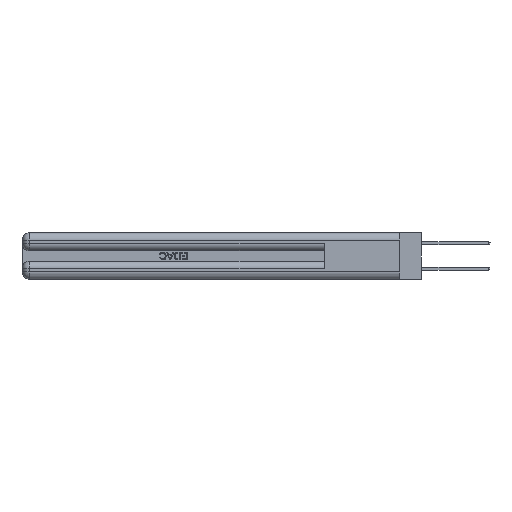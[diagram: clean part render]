
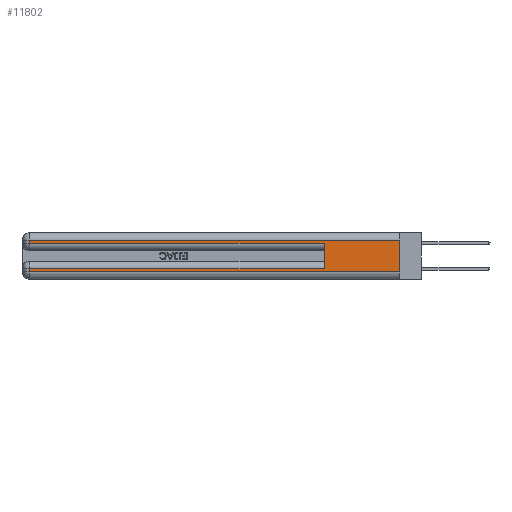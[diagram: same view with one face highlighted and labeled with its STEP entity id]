
A CAD part, left-side view. The second image highlights one B-rep face of the part: STEP entity #11802.
In plain terms, the highlighted planar face has unit normal (-1, 0, 0).
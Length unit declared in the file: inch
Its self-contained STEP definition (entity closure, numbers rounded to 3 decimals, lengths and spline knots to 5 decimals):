
#711 = DIRECTION ( 'NONE',  ( 0., -1., 0. ) ) ;
#1055 = VECTOR ( 'NONE', #711, 39.37008 ) ;
#1711 = EDGE_CURVE ( 'NONE', #34496, #46931, #38199, .T. ) ;
#2242 = DIRECTION ( 'NONE',  ( 1., 0., 0. ) ) ;
#2792 = VERTEX_POINT ( 'NONE', #23852 ) ;
#2886 = DIRECTION ( 'NONE',  ( 0., -1., 0. ) ) ;
#3246 = ORIENTED_EDGE ( 'NONE', *, *, #6224, .T. ) ;
#3574 = EDGE_CURVE ( 'NONE', #2792, #42154, #43149, .T. ) ;
#4545 = LINE ( 'NONE', #44220, #30268 ) ;
#6024 = CARTESIAN_POINT ( 'NONE',  ( 0., 0.6, 0.145 ) ) ;
#6224 = EDGE_CURVE ( 'NONE', #8268, #46931, #25648, .T. ) ;
#7801 = VECTOR ( 'NONE', #20749, 39.37008 ) ;
#8268 = VERTEX_POINT ( 'NONE', #28510 ) ;
#10424 = EDGE_LOOP ( 'NONE', ( #37490, #43085, #34774, #3246, #31566, #31514, #31092, #27374 ) ) ;
#10756 = CARTESIAN_POINT ( 'NONE',  ( 0., 2.94, 0.085 ) ) ;
#11802 = ADVANCED_FACE ( 'NONE', ( #24345 ), #24091, .F. ) ;
#12672 = VERTEX_POINT ( 'NONE', #22584 ) ;
#13892 = VECTOR ( 'NONE', #20384, 39.37008 ) ;
#14137 = VECTOR ( 'NONE', #45465, 39.37008 ) ;
#15295 = LINE ( 'NONE', #41638, #14137 ) ;
#15775 = VECTOR ( 'NONE', #31794, 39.37008 ) ;
#15935 = VECTOR ( 'NONE', #2886, 39.37008 ) ;
#18915 = CARTESIAN_POINT ( 'NONE',  ( 0., 0., 0.06 ) ) ;
#20384 = DIRECTION ( 'NONE',  ( 0., 1., 0. ) ) ;
#20749 = DIRECTION ( 'NONE',  ( 0., 0., 1. ) ) ;
#22584 = CARTESIAN_POINT ( 'NONE',  ( 0., 2.94, 0.06 ) ) ;
#22825 = EDGE_CURVE ( 'NONE', #42154, #8268, #15295, .T. ) ;
#23852 = CARTESIAN_POINT ( 'NONE',  ( 0., 0., 0.31 ) ) ;
#24046 = CARTESIAN_POINT ( 'NONE',  ( 0., 0., 0.31 ) ) ;
#24083 = CARTESIAN_POINT ( 'NONE',  ( 0., 0., 0.06 ) ) ;
#24091 = PLANE ( 'NONE',  #29608 ) ;
#24345 = FACE_OUTER_BOUND ( 'NONE', #10424, .T. ) ;
#25014 = CARTESIAN_POINT ( 'NONE',  ( 0., 0.6, 0.285 ) ) ;
#25648 = LINE ( 'NONE', #28411, #15935 ) ;
#27370 = EDGE_CURVE ( 'NONE', #34496, #30808, #35233, .T. ) ;
#27374 = ORIENTED_EDGE ( 'NONE', *, *, #32961, .T. ) ;
#27759 = DIRECTION ( 'NONE',  ( 0., 0., -1. ) ) ;
#28119 = CARTESIAN_POINT ( 'NONE',  ( 0., 0., 0.085 ) ) ;
#28411 = CARTESIAN_POINT ( 'NONE',  ( 0., 0., 0.285 ) ) ;
#28510 = CARTESIAN_POINT ( 'NONE',  ( 0., 2.94, 0.285 ) ) ;
#28837 = CARTESIAN_POINT ( 'NONE',  ( 0., 2.94, 0.37 ) ) ;
#29608 = AXIS2_PLACEMENT_3D ( 'NONE', #46058, #2242, #27759 ) ;
#29613 = DIRECTION ( 'NONE',  ( 0., 0., -1. ) ) ;
#29888 = VERTEX_POINT ( 'NONE', #24083 ) ;
#30268 = VECTOR ( 'NONE', #29613, 39.37008 ) ;
#30808 = VERTEX_POINT ( 'NONE', #10756 ) ;
#30869 = EDGE_CURVE ( 'NONE', #2792, #29888, #4545, .T. ) ;
#31092 = ORIENTED_EDGE ( 'NONE', *, *, #46972, .T. ) ;
#31514 = ORIENTED_EDGE ( 'NONE', *, *, #27370, .T. ) ;
#31566 = ORIENTED_EDGE ( 'NONE', *, *, #1711, .F. ) ;
#31794 = DIRECTION ( 'NONE',  ( 0., 1., 0. ) ) ;
#32542 = DIRECTION ( 'NONE',  ( 0., 0., -1. ) ) ;
#32790 = LINE ( 'NONE', #28837, #41438 ) ;
#32961 = EDGE_CURVE ( 'NONE', #12672, #29888, #38835, .T. ) ;
#34496 = VERTEX_POINT ( 'NONE', #37695 ) ;
#34774 = ORIENTED_EDGE ( 'NONE', *, *, #22825, .T. ) ;
#35233 = LINE ( 'NONE', #28119, #15775 ) ;
#37490 = ORIENTED_EDGE ( 'NONE', *, *, #30869, .F. ) ;
#37695 = CARTESIAN_POINT ( 'NONE',  ( 0., 0.6, 0.085 ) ) ;
#38199 = LINE ( 'NONE', #6024, #7801 ) ;
#38835 = LINE ( 'NONE', #18915, #1055 ) ;
#41438 = VECTOR ( 'NONE', #32542, 39.37008 ) ;
#41638 = CARTESIAN_POINT ( 'NONE',  ( 0., 2.94, 0.37 ) ) ;
#42154 = VERTEX_POINT ( 'NONE', #47356 ) ;
#43085 = ORIENTED_EDGE ( 'NONE', *, *, #3574, .T. ) ;
#43149 = LINE ( 'NONE', #24046, #13892 ) ;
#44220 = CARTESIAN_POINT ( 'NONE',  ( 0., 0., 0.37 ) ) ;
#45465 = DIRECTION ( 'NONE',  ( 0., 0., -1. ) ) ;
#46058 = CARTESIAN_POINT ( 'NONE',  ( 0., 0., 0.37 ) ) ;
#46931 = VERTEX_POINT ( 'NONE', #25014 ) ;
#46972 = EDGE_CURVE ( 'NONE', #30808, #12672, #32790, .T. ) ;
#47356 = CARTESIAN_POINT ( 'NONE',  ( 0., 2.94, 0.31 ) ) ;
